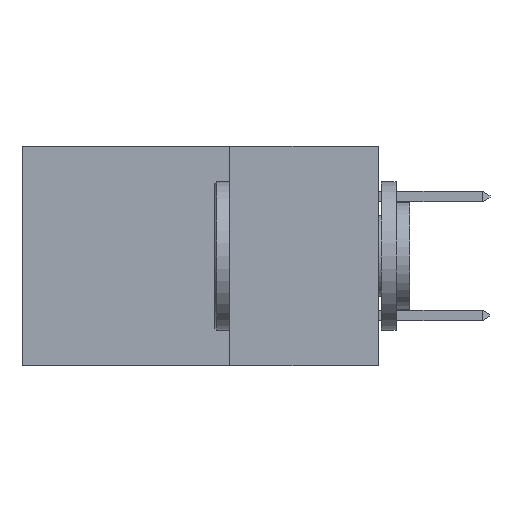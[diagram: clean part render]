
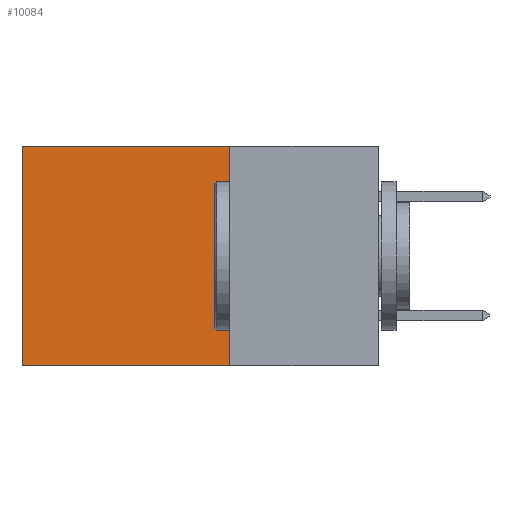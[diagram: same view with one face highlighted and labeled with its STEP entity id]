
A CAD part, left-side view. The second image highlights one B-rep face of the part: STEP entity #10084.
In plain terms, the highlighted planar face has unit normal (-1, 0, 0).
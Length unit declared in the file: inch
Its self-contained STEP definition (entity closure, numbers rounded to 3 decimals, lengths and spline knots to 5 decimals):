
#420 = ORIENTED_EDGE ( 'NONE', *, *, #15307, .T. ) ;
#919 = CARTESIAN_POINT ( 'NONE',  ( 0.298, 0.25, -0.37 ) ) ;
#1065 = CARTESIAN_POINT ( 'NONE',  ( 0.298, 0.25, 0. ) ) ;
#1229 = VECTOR ( 'NONE', #4566, 39.37008 ) ;
#1934 = ORIENTED_EDGE ( 'NONE', *, *, #23226, .F. ) ;
#1963 = VECTOR ( 'NONE', #17668, 39.37008 ) ;
#2751 = VECTOR ( 'NONE', #13905, 39.37008 ) ;
#4566 = DIRECTION ( 'NONE',  ( 0., 1., 0. ) ) ;
#5058 = VERTEX_POINT ( 'NONE', #6730 ) ;
#5425 = PLANE ( 'NONE',  #19997 ) ;
#6074 = LINE ( 'NONE', #919, #1229 ) ;
#6596 = CARTESIAN_POINT ( 'NONE',  ( 0.298, 0.25, 0. ) ) ;
#6730 = CARTESIAN_POINT ( 'NONE',  ( 0.298, 0.6, 0. ) ) ;
#7212 = LINE ( 'NONE', #9144, #11534 ) ;
#7288 = DIRECTION ( 'NONE',  ( 0., 0., -1. ) ) ;
#9144 = CARTESIAN_POINT ( 'NONE',  ( 0.298, 0.6, 0. ) ) ;
#9434 = EDGE_LOOP ( 'NONE', ( #12938, #14423, #1934, #420 ) ) ;
#10084 = ADVANCED_FACE ( 'NONE', ( #20503 ), #5425, .F. ) ;
#10588 = CARTESIAN_POINT ( 'NONE',  ( 0.298, 0.25, -0.37 ) ) ;
#11534 = VECTOR ( 'NONE', #16522, 39.37008 ) ;
#11740 = CARTESIAN_POINT ( 'NONE',  ( 0.298, 0.25, 0. ) ) ;
#12445 = CARTESIAN_POINT ( 'NONE',  ( 0.298, 0.25, 0. ) ) ;
#12845 = EDGE_CURVE ( 'NONE', #23566, #21610, #6074, .T. ) ;
#12938 = ORIENTED_EDGE ( 'NONE', *, *, #13268, .T. ) ;
#13268 = EDGE_CURVE ( 'NONE', #5058, #21610, #7212, .T. ) ;
#13905 = DIRECTION ( 'NONE',  ( 0., 0., -1. ) ) ;
#14423 = ORIENTED_EDGE ( 'NONE', *, *, #12845, .F. ) ;
#14937 = CARTESIAN_POINT ( 'NONE',  ( 0.298, 0.6, -0.37 ) ) ;
#15307 = EDGE_CURVE ( 'NONE', #23151, #5058, #21419, .T. ) ;
#16522 = DIRECTION ( 'NONE',  ( 0., 0., -1. ) ) ;
#16796 = LINE ( 'NONE', #1065, #2751 ) ;
#17668 = DIRECTION ( 'NONE',  ( 0., 1., 0. ) ) ;
#18295 = DIRECTION ( 'NONE',  ( 1., 0., 0. ) ) ;
#19997 = AXIS2_PLACEMENT_3D ( 'NONE', #12445, #18295, #7288 ) ;
#20503 = FACE_OUTER_BOUND ( 'NONE', #9434, .T. ) ;
#21419 = LINE ( 'NONE', #6596, #1963 ) ;
#21610 = VERTEX_POINT ( 'NONE', #14937 ) ;
#23151 = VERTEX_POINT ( 'NONE', #11740 ) ;
#23226 = EDGE_CURVE ( 'NONE', #23151, #23566, #16796, .T. ) ;
#23566 = VERTEX_POINT ( 'NONE', #10588 ) ;
